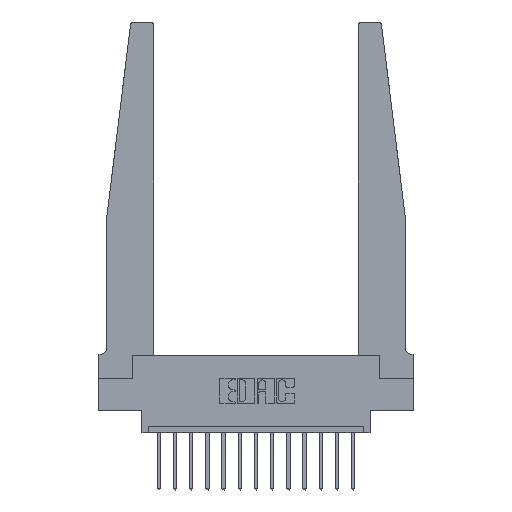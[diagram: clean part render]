
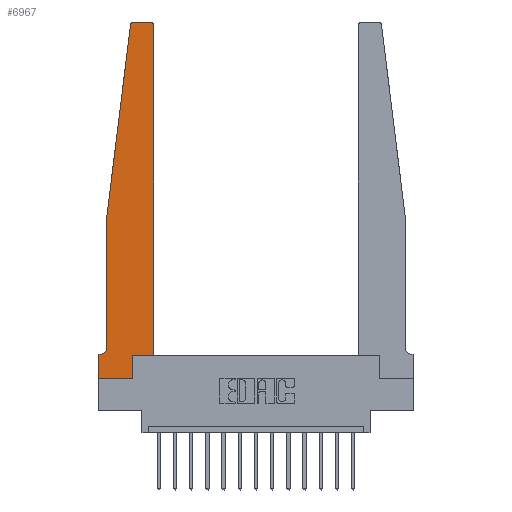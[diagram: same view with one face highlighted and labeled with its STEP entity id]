
A CAD part, top view. The second image highlights one B-rep face of the part: STEP entity #6967.
In plain terms, the highlighted planar face has unit normal (0, 0, 1).
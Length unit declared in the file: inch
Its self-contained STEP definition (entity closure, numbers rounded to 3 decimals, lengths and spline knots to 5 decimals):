
#123 = VERTEX_POINT ( 'NONE', #5915 ) ;
#155 = VERTEX_POINT ( 'NONE', #9870 ) ;
#180 = DIRECTION ( 'NONE',  ( -1., 0., 0. ) ) ;
#369 = CARTESIAN_POINT ( 'NONE',  ( 0.395, 2.75, 0.37 ) ) ;
#415 = CIRCLE ( 'NONE', #10505, 0.03 ) ;
#442 = VERTEX_POINT ( 'NONE', #14368 ) ;
#451 = AXIS2_PLACEMENT_3D ( 'NONE', #2376, #13096, #1062 ) ;
#467 = CARTESIAN_POINT ( 'NONE',  ( 0., 0., 0.37 ) ) ;
#726 = VECTOR ( 'NONE', #10112, 39.37008 ) ;
#748 = VECTOR ( 'NONE', #1219, 39.37008 ) ;
#1062 = DIRECTION ( 'NONE',  ( -1., 0., 0. ) ) ;
#1219 = DIRECTION ( 'NONE',  ( -1., 0., 0. ) ) ;
#1245 = DIRECTION ( 'NONE',  ( 0., 1., 0. ) ) ;
#1502 = CARTESIAN_POINT ( 'NONE',  ( 0.25, 2.75, 0.37 ) ) ;
#1520 = CARTESIAN_POINT ( 'NONE',  ( 0., 0.1875, 0.37 ) ) ;
#1735 = VERTEX_POINT ( 'NONE', #5740 ) ;
#1764 = VERTEX_POINT ( 'NONE', #5558 ) ;
#1833 = CARTESIAN_POINT ( 'NONE',  ( 0.27653, 2.72, 0.37 ) ) ;
#1909 = ORIENTED_EDGE ( 'NONE', *, *, #4122, .T. ) ;
#2376 = CARTESIAN_POINT ( 'NONE',  ( 0.015, 0.2375, 0.37 ) ) ;
#2425 = EDGE_CURVE ( 'NONE', #1735, #1764, #15709, .T. ) ;
#2676 = CARTESIAN_POINT ( 'NONE',  ( 0.065, 1.25, 0.37 ) ) ;
#2913 = VERTEX_POINT ( 'NONE', #13250 ) ;
#3251 = CARTESIAN_POINT ( 'NONE',  ( 0.2605, 0., 0.37 ) ) ;
#3324 = VERTEX_POINT ( 'NONE', #467 ) ;
#3331 = EDGE_CURVE ( 'NONE', #13854, #2913, #14712, .T. ) ;
#3507 = LINE ( 'NONE', #7289, #726 ) ;
#3924 = VECTOR ( 'NONE', #1245, 39.37008 ) ;
#4122 = EDGE_CURVE ( 'NONE', #16801, #13854, #8470, .T. ) ;
#4178 = EDGE_CURVE ( 'NONE', #15344, #123, #9467, .T. ) ;
#4239 = FACE_OUTER_BOUND ( 'NONE', #10165, .T. ) ;
#4426 = CARTESIAN_POINT ( 'NONE',  ( 0., 0., 0.37 ) ) ;
#4490 = PLANE ( 'NONE',  #11058 ) ;
#4662 = CARTESIAN_POINT ( 'NONE',  ( 0., 0., 0.37 ) ) ;
#4799 = CARTESIAN_POINT ( 'NONE',  ( 0.24675, 2.72367, 0.37 ) ) ;
#5140 = ORIENTED_EDGE ( 'NONE', *, *, #9924, .T. ) ;
#5292 = EDGE_CURVE ( 'NONE', #3324, #15344, #16426, .T. ) ;
#5331 = ORIENTED_EDGE ( 'NONE', *, *, #8844, .T. ) ;
#5372 = DIRECTION ( 'NONE',  ( 1., 0., 0. ) ) ;
#5558 = CARTESIAN_POINT ( 'NONE',  ( 0.425, 2.72, 0.37 ) ) ;
#5668 = ORIENTED_EDGE ( 'NONE', *, *, #9421, .T. ) ;
#5740 = CARTESIAN_POINT ( 'NONE',  ( 0.425, 0.18, 0.37 ) ) ;
#5915 = CARTESIAN_POINT ( 'NONE',  ( 0.2605, 0.18, 0.37 ) ) ;
#6499 = ORIENTED_EDGE ( 'NONE', *, *, #13634, .T. ) ;
#6658 = DIRECTION ( 'NONE',  ( 0., 1., 0. ) ) ;
#6889 = DIRECTION ( 'NONE',  ( 0., 0., 1. ) ) ;
#6967 = ADVANCED_FACE ( 'NONE', ( #4239 ), #4490, .T. ) ;
#6969 = LINE ( 'NONE', #4662, #17025 ) ;
#7218 = DIRECTION ( 'NONE',  ( 1., 0., 0. ) ) ;
#7289 = CARTESIAN_POINT ( 'NONE',  ( 0.425, 0.18, 0.37 ) ) ;
#7617 = LINE ( 'NONE', #10257, #748 ) ;
#7737 = EDGE_CURVE ( 'NONE', #442, #16801, #415, .T. ) ;
#8104 = ORIENTED_EDGE ( 'NONE', *, *, #4178, .T. ) ;
#8395 = DIRECTION ( 'NONE',  ( 1., 0., 0. ) ) ;
#8470 = LINE ( 'NONE', #16191, #11040 ) ;
#8654 = ORIENTED_EDGE ( 'NONE', *, *, #7737, .T. ) ;
#8786 = VECTOR ( 'NONE', #8395, 39.37008 ) ;
#8844 = EDGE_CURVE ( 'NONE', #123, #1735, #3507, .T. ) ;
#8998 = EDGE_CURVE ( 'NONE', #2913, #155, #9975, .T. ) ;
#9421 = EDGE_CURVE ( 'NONE', #155, #15131, #7617, .T. ) ;
#9467 = LINE ( 'NONE', #13336, #13386 ) ;
#9870 = CARTESIAN_POINT ( 'NONE',  ( 0.015, 0.1875, 0.37 ) ) ;
#9924 = EDGE_CURVE ( 'NONE', #1764, #15251, #16980, .T. ) ;
#9975 = CIRCLE ( 'NONE', #451, 0.05 ) ;
#10112 = DIRECTION ( 'NONE',  ( 1., 0., 0. ) ) ;
#10165 = EDGE_LOOP ( 'NONE', ( #16033, #8654, #1909, #14774, #13245, #5668, #6499, #11224, #8104, #5331, #11720, #5140 ) ) ;
#10257 = CARTESIAN_POINT ( 'NONE',  ( 0.065, 0.1875, 0.37 ) ) ;
#10274 = AXIS2_PLACEMENT_3D ( 'NONE', #13652, #6889, #5372 ) ;
#10347 = EDGE_CURVE ( 'NONE', #15251, #442, #16462, .T. ) ;
#10505 = AXIS2_PLACEMENT_3D ( 'NONE', #1833, #14918, #12553 ) ;
#10869 = DIRECTION ( 'NONE',  ( -0.122, -0.992, 0. ) ) ;
#11040 = VECTOR ( 'NONE', #10869, 39.37008 ) ;
#11058 = AXIS2_PLACEMENT_3D ( 'NONE', #15127, #13908, #7218 ) ;
#11224 = ORIENTED_EDGE ( 'NONE', *, *, #5292, .T. ) ;
#11720 = ORIENTED_EDGE ( 'NONE', *, *, #2425, .T. ) ;
#12553 = DIRECTION ( 'NONE',  ( 1., 0., 0. ) ) ;
#12678 = DIRECTION ( 'NONE',  ( 0., -1., 0. ) ) ;
#13096 = DIRECTION ( 'NONE',  ( 0., 0., -1. ) ) ;
#13245 = ORIENTED_EDGE ( 'NONE', *, *, #8998, .T. ) ;
#13250 = CARTESIAN_POINT ( 'NONE',  ( 0.065, 0.2375, 0.37 ) ) ;
#13336 = CARTESIAN_POINT ( 'NONE',  ( 0.2605, 0.18, 0.37 ) ) ;
#13386 = VECTOR ( 'NONE', #6658, 39.37008 ) ;
#13634 = EDGE_CURVE ( 'NONE', #15131, #3324, #6969, .T. ) ;
#13652 = CARTESIAN_POINT ( 'NONE',  ( 0.395, 2.72, 0.37 ) ) ;
#13854 = VERTEX_POINT ( 'NONE', #16769 ) ;
#13908 = DIRECTION ( 'NONE',  ( 0., 0., 1. ) ) ;
#14368 = CARTESIAN_POINT ( 'NONE',  ( 0.27653, 2.75, 0.37 ) ) ;
#14627 = DIRECTION ( 'NONE',  ( 0., -1., 0. ) ) ;
#14712 = LINE ( 'NONE', #2676, #16581 ) ;
#14774 = ORIENTED_EDGE ( 'NONE', *, *, #3331, .T. ) ;
#14918 = DIRECTION ( 'NONE',  ( 0., 0., 1. ) ) ;
#15127 = CARTESIAN_POINT ( 'NONE',  ( 0., 0.1875, 0.37 ) ) ;
#15131 = VERTEX_POINT ( 'NONE', #1520 ) ;
#15251 = VERTEX_POINT ( 'NONE', #369 ) ;
#15344 = VERTEX_POINT ( 'NONE', #3251 ) ;
#15709 = LINE ( 'NONE', #17185, #3924 ) ;
#16033 = ORIENTED_EDGE ( 'NONE', *, *, #10347, .T. ) ;
#16191 = CARTESIAN_POINT ( 'NONE',  ( 0.065, 1.25, 0.37 ) ) ;
#16426 = LINE ( 'NONE', #4426, #8786 ) ;
#16462 = LINE ( 'NONE', #1502, #16993 ) ;
#16581 = VECTOR ( 'NONE', #14627, 39.37008 ) ;
#16769 = CARTESIAN_POINT ( 'NONE',  ( 0.065, 1.25, 0.37 ) ) ;
#16801 = VERTEX_POINT ( 'NONE', #4799 ) ;
#16980 = CIRCLE ( 'NONE', #10274, 0.03 ) ;
#16993 = VECTOR ( 'NONE', #180, 39.37008 ) ;
#17025 = VECTOR ( 'NONE', #12678, 39.37008 ) ;
#17185 = CARTESIAN_POINT ( 'NONE',  ( 0.425, 0.18, 0.37 ) ) ;
